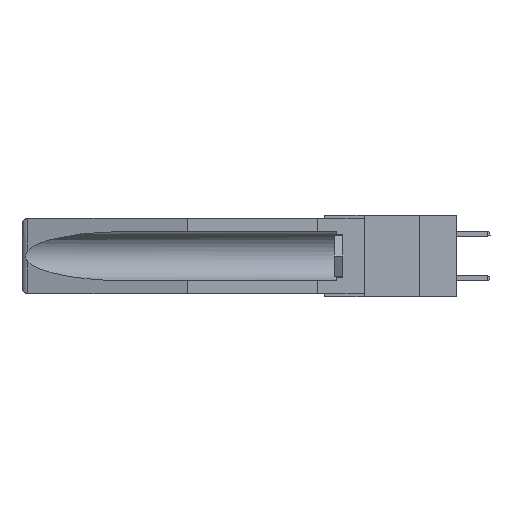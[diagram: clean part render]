
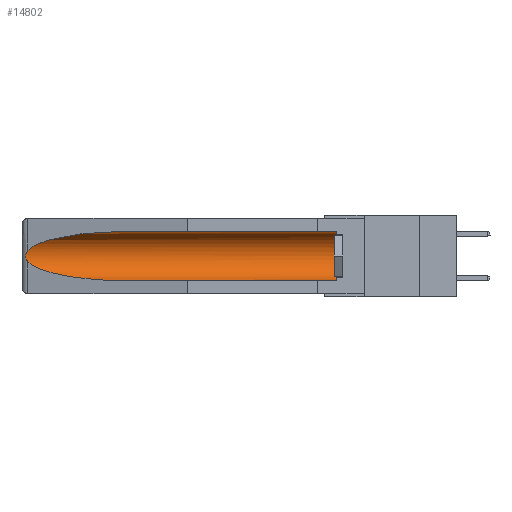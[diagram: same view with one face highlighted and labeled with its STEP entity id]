
A CAD part, left-side view. The second image highlights one B-rep face of the part: STEP entity #14802.
In plain terms, the highlighted cylindrical face has radius 2.857 mm (diameter 5.715 mm), a partial arc.
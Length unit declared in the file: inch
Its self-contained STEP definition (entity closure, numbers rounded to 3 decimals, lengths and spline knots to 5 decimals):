
#190 = LINE ( 'NONE', #10775, #3440 ) ;
#747 = CARTESIAN_POINT ( 'NONE',  ( 0.2675, 1.53308, -0.17534 ) ) ;
#914 = DIRECTION ( 'NONE',  ( 0., 0., 1. ) ) ;
#920 = CARTESIAN_POINT ( 'NONE',  ( 0.25451, 1.48313, -0.09465 ) ) ;
#1563 = CARTESIAN_POINT ( 'NONE',  ( 0.155, 0.126, -0.1715 ) ) ;
#2819 = DIRECTION ( 'NONE',  ( 0., 1., 0. ) ) ;
#3138 = VERTEX_POINT ( 'NONE', #5835 ) ;
#3151 = CARTESIAN_POINT ( 'NONE',  ( 0.2673, 1.5327, -0.16383 ) ) ;
#3256 = CARTESIAN_POINT ( 'NONE',  ( 0.26537, 1.52718, -0.19328 ) ) ;
#3440 = VECTOR ( 'NONE', #29371, 39.37008 ) ;
#4766 =( BOUNDED_CURVE ( )  B_SPLINE_CURVE ( 3, ( #20389, #25360, #15645, #6548 ),
 .UNSPECIFIED., .F., .F. ) 
 B_SPLINE_CURVE_WITH_KNOTS ( ( 4, 4 ),
 ( 0.1948, 1.5708 ),
 .UNSPECIFIED. ) 
 CURVE ( )  GEOMETRIC_REPRESENTATION_ITEM ( )  RATIONAL_B_SPLINE_CURVE ( ( 1., 0.848, 0.848, 1. ) ) 
 REPRESENTATION_ITEM ( '' )  );
#5508 = CARTESIAN_POINT ( 'NONE',  ( 0.26597, 1.5296, -0.19026 ) ) ;
#5788 = CARTESIAN_POINT ( 'NONE',  ( 0.155, 1.07973, -0.059 ) ) ;
#5835 = CARTESIAN_POINT ( 'NONE',  ( 0.155, 1.07973, -0.284 ) ) ;
#6548 = CARTESIAN_POINT ( 'NONE',  ( 0.155, 1.07973, -0.284 ) ) ;
#7560 = B_SPLINE_CURVE_WITH_KNOTS ( 'NONE', 3,
 ( #12209, #21482, #14611, #3151, #7847, #747, #9866, #12115, #5508, #3256 ),
 .UNSPECIFIED., .F., .F.,
 ( 4, 2, 2, 2, 4 ),
 ( 0., 0.00029, 0.00058, 0.00087, 0.00117 ),
 .UNSPECIFIED. ) ;
#7712 = CARTESIAN_POINT ( 'NONE',  ( 0.26537, 1.52718, -0.14972 ) ) ;
#7847 = CARTESIAN_POINT ( 'NONE',  ( 0.2675, 1.53308, -0.16763 ) ) ;
#8040 = VERTEX_POINT ( 'NONE', #12797 ) ;
#8116 = CARTESIAN_POINT ( 'NONE',  ( 0.21114, 1.30732, -0.059 ) ) ;
#8963 = ORIENTED_EDGE ( 'NONE', *, *, #26169, .F. ) ;
#8970 = AXIS2_PLACEMENT_3D ( 'NONE', #21739, #2819, #914 ) ;
#9296 = ORIENTED_EDGE ( 'NONE', *, *, #22812, .T. ) ;
#9530 = CARTESIAN_POINT ( 'NONE',  ( 0.155, 0.126, -0.059 ) ) ;
#9774 = EDGE_CURVE ( 'NONE', #10484, #24993, #26850, .T. ) ;
#9866 = CARTESIAN_POINT ( 'NONE',  ( 0.2673, 1.53269, -0.17917 ) ) ;
#10430 = AXIS2_PLACEMENT_3D ( 'NONE', #1563, #15850, #13441 ) ;
#10484 = VERTEX_POINT ( 'NONE', #9530 ) ;
#10663 = CYLINDRICAL_SURFACE ( 'NONE', #8970, 0.1125 ) ;
#10775 = CARTESIAN_POINT ( 'NONE',  ( 0.155, -0.30754, -0.284 ) ) ;
#11394 = VERTEX_POINT ( 'NONE', #21375 ) ;
#12115 = CARTESIAN_POINT ( 'NONE',  ( 0.26655, 1.53094, -0.18657 ) ) ;
#12209 = CARTESIAN_POINT ( 'NONE',  ( 0.26537, 1.52718, -0.14972 ) ) ;
#12797 = CARTESIAN_POINT ( 'NONE',  ( 0.26537, 1.52718, -0.19328 ) ) ;
#13414 = VERTEX_POINT ( 'NONE', #27091 ) ;
#13441 = DIRECTION ( 'NONE',  ( 0., 0., 1. ) ) ;
#14611 = CARTESIAN_POINT ( 'NONE',  ( 0.26654, 1.53092, -0.15636 ) ) ;
#14802 = ADVANCED_FACE ( 'NONE', ( #21125 ), #10663, .F. ) ;
#15398 = ORIENTED_EDGE ( 'NONE', *, *, #28172, .T. ) ;
#15645 = CARTESIAN_POINT ( 'NONE',  ( 0.21114, 1.30732, -0.284 ) ) ;
#15850 = DIRECTION ( 'NONE',  ( 0., -1., 0. ) ) ;
#15874 = CARTESIAN_POINT ( 'NONE',  ( 0.155, -0.30754, -0.059 ) ) ;
#15938 = CIRCLE ( 'NONE', #10430, 0.1125 ) ;
#16886 = ORIENTED_EDGE ( 'NONE', *, *, #23453, .T. ) ;
#18299 =( BOUNDED_CURVE ( )  B_SPLINE_CURVE ( 3, ( #5788, #8116, #920, #7712 ),
 .UNSPECIFIED., .F., .F. ) 
 B_SPLINE_CURVE_WITH_KNOTS ( ( 4, 4 ),
 ( 4.71239, 6.08839 ),
 .UNSPECIFIED. ) 
 CURVE ( )  GEOMETRIC_REPRESENTATION_ITEM ( )  RATIONAL_B_SPLINE_CURVE ( ( 1., 0.848, 0.848, 1. ) ) 
 REPRESENTATION_ITEM ( '' )  );
#20225 = DIRECTION ( 'NONE',  ( 0., 1., 0. ) ) ;
#20389 = CARTESIAN_POINT ( 'NONE',  ( 0.26537, 1.52718, -0.19328 ) ) ;
#21125 = FACE_OUTER_BOUND ( 'NONE', #27939, .T. ) ;
#21375 = CARTESIAN_POINT ( 'NONE',  ( 0.26537, 1.52718, -0.14972 ) ) ;
#21482 = CARTESIAN_POINT ( 'NONE',  ( 0.26597, 1.52961, -0.15275 ) ) ;
#21697 = ORIENTED_EDGE ( 'NONE', *, *, #28868, .T. ) ;
#21739 = CARTESIAN_POINT ( 'NONE',  ( 0.155, -0.30754, -0.1715 ) ) ;
#22237 = ORIENTED_EDGE ( 'NONE', *, *, #9774, .T. ) ;
#22812 = EDGE_CURVE ( 'NONE', #13414, #10484, #15938, .T. ) ;
#23453 = EDGE_CURVE ( 'NONE', #24993, #11394, #18299, .T. ) ;
#24993 = VERTEX_POINT ( 'NONE', #28854 ) ;
#25360 = CARTESIAN_POINT ( 'NONE',  ( 0.25451, 1.48313, -0.24835 ) ) ;
#26169 = EDGE_CURVE ( 'NONE', #13414, #3138, #190, .T. ) ;
#26850 = LINE ( 'NONE', #15874, #27227 ) ;
#27091 = CARTESIAN_POINT ( 'NONE',  ( 0.155, 0.126, -0.284 ) ) ;
#27227 = VECTOR ( 'NONE', #20225, 39.37008 ) ;
#27939 = EDGE_LOOP ( 'NONE', ( #16886, #21697, #15398, #8963, #9296, #22237 ) ) ;
#28172 = EDGE_CURVE ( 'NONE', #8040, #3138, #4766, .T. ) ;
#28854 = CARTESIAN_POINT ( 'NONE',  ( 0.155, 1.07973, -0.059 ) ) ;
#28868 = EDGE_CURVE ( 'NONE', #11394, #8040, #7560, .T. ) ;
#29371 = DIRECTION ( 'NONE',  ( 0., 1., 0. ) ) ;
